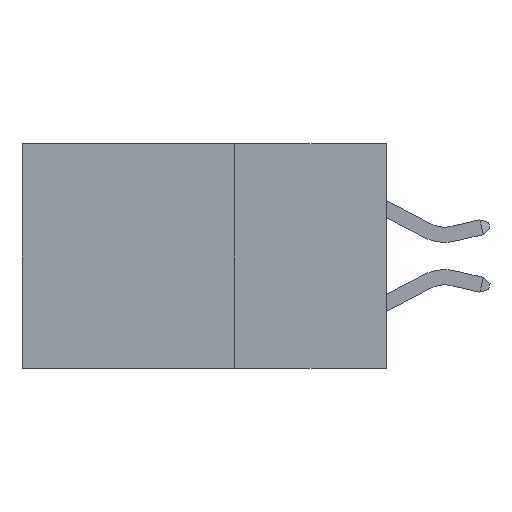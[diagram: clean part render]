
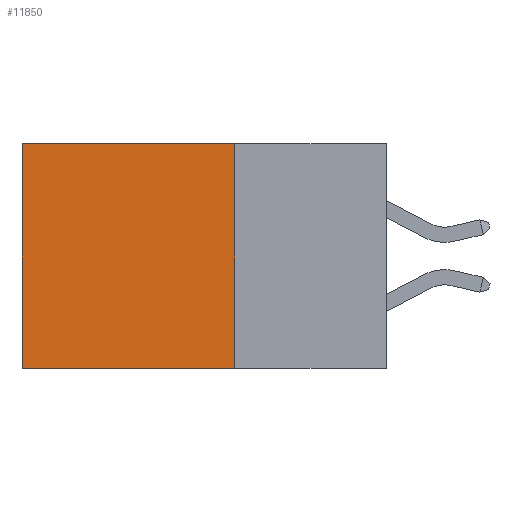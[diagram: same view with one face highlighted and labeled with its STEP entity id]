
A CAD part, left-side view. The second image highlights one B-rep face of the part: STEP entity #11850.
In plain terms, the highlighted planar face has unit normal (-1, 0, 0).
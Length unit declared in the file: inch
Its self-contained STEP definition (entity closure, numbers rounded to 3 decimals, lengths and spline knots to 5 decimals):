
#21 = EDGE_CURVE ( 'NONE', #5078, #4344, #880, .T. ) ;
#138 = EDGE_CURVE ( 'NONE', #8342, #6799, #12048, .T. ) ;
#338 = CARTESIAN_POINT ( 'NONE',  ( 0.2615, 0.25, -0.37 ) ) ;
#426 = DIRECTION ( 'NONE',  ( 0., 0., -1. ) ) ;
#634 = VECTOR ( 'NONE', #2789, 39.37008 ) ;
#880 = LINE ( 'NONE', #11351, #6065 ) ;
#1128 = VECTOR ( 'NONE', #8372, 39.37008 ) ;
#1661 = DIRECTION ( 'NONE',  ( 0., 0., -1. ) ) ;
#1799 = EDGE_CURVE ( 'NONE', #8342, #5078, #3965, .T. ) ;
#2789 = DIRECTION ( 'NONE',  ( 0., 1., 0. ) ) ;
#3638 = EDGE_LOOP ( 'NONE', ( #8331, #12099, #11488, #12156 ) ) ;
#3757 = EDGE_CURVE ( 'NONE', #6799, #4344, #9125, .T. ) ;
#3965 = LINE ( 'NONE', #9969, #1128 ) ;
#4344 = VERTEX_POINT ( 'NONE', #11242 ) ;
#4892 = CARTESIAN_POINT ( 'NONE',  ( 0.2615, 0.25, -0.37 ) ) ;
#5078 = VERTEX_POINT ( 'NONE', #7576 ) ;
#6065 = VECTOR ( 'NONE', #426, 39.37008 ) ;
#6537 = AXIS2_PLACEMENT_3D ( 'NONE', #6793, #9745, #1661 ) ;
#6619 = FACE_OUTER_BOUND ( 'NONE', #3638, .T. ) ;
#6793 = CARTESIAN_POINT ( 'NONE',  ( 0.2615, 0.25, -0.37 ) ) ;
#6799 = VERTEX_POINT ( 'NONE', #10300 ) ;
#7576 = CARTESIAN_POINT ( 'NONE',  ( 0.2615, 0.6, 0. ) ) ;
#7788 = PLANE ( 'NONE',  #6537 ) ;
#8331 = ORIENTED_EDGE ( 'NONE', *, *, #21, .T. ) ;
#8342 = VERTEX_POINT ( 'NONE', #10741 ) ;
#8372 = DIRECTION ( 'NONE',  ( 0., 1., 0. ) ) ;
#9125 = LINE ( 'NONE', #4892, #634 ) ;
#9745 = DIRECTION ( 'NONE',  ( 1., 0., 0. ) ) ;
#9969 = CARTESIAN_POINT ( 'NONE',  ( 0.2615, 0.25, 0. ) ) ;
#10300 = CARTESIAN_POINT ( 'NONE',  ( 0.2615, 0.25, -0.37 ) ) ;
#10741 = CARTESIAN_POINT ( 'NONE',  ( 0.2615, 0.25, 0. ) ) ;
#11242 = CARTESIAN_POINT ( 'NONE',  ( 0.2615, 0.6, -0.37 ) ) ;
#11351 = CARTESIAN_POINT ( 'NONE',  ( 0.2615, 0.6, -0.37 ) ) ;
#11477 = VECTOR ( 'NONE', #12176, 39.37008 ) ;
#11488 = ORIENTED_EDGE ( 'NONE', *, *, #138, .F. ) ;
#11850 = ADVANCED_FACE ( 'NONE', ( #6619 ), #7788, .F. ) ;
#12048 = LINE ( 'NONE', #338, #11477 ) ;
#12099 = ORIENTED_EDGE ( 'NONE', *, *, #3757, .F. ) ;
#12156 = ORIENTED_EDGE ( 'NONE', *, *, #1799, .T. ) ;
#12176 = DIRECTION ( 'NONE',  ( 0., 0., -1. ) ) ;
